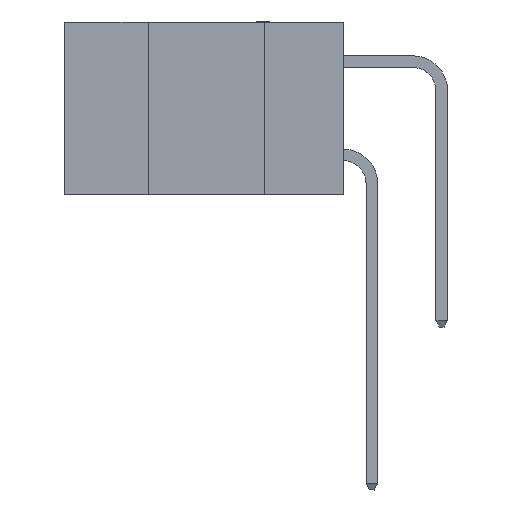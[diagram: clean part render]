
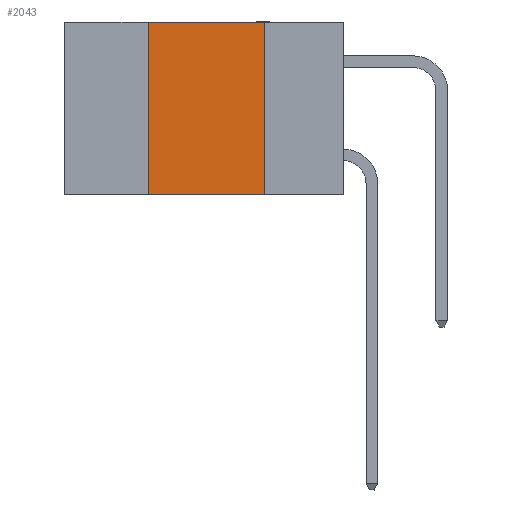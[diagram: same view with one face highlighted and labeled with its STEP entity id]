
A CAD part, left-side view. The second image highlights one B-rep face of the part: STEP entity #2043.
In plain terms, the highlighted planar face has unit normal (-1, 0, 0).
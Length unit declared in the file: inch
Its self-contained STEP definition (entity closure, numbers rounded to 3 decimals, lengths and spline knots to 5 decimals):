
#1115 = ORIENTED_EDGE ( 'NONE', *, *, #20038, .T. ) ;
#1782 = VECTOR ( 'NONE', #17318, 39.37008 ) ;
#2043 = ADVANCED_FACE ( 'NONE', ( #27690 ), #28479, .F. ) ;
#3491 = EDGE_CURVE ( 'NONE', #28054, #3561, #6715, .T. ) ;
#3561 = VERTEX_POINT ( 'NONE', #16564 ) ;
#5128 = VECTOR ( 'NONE', #19442, 39.37008 ) ;
#5188 = CARTESIAN_POINT ( 'NONE',  ( 0., 0.42, 0. ) ) ;
#5946 = DIRECTION ( 'NONE',  ( 0., 0., -1. ) ) ;
#6048 = DIRECTION ( 'NONE',  ( 1., 0., 0. ) ) ;
#6220 = DIRECTION ( 'NONE',  ( 0., -1., 0. ) ) ;
#6502 = VECTOR ( 'NONE', #22907, 39.37008 ) ;
#6715 = LINE ( 'NONE', #16647, #5128 ) ;
#7099 = ORIENTED_EDGE ( 'NONE', *, *, #25659, .F. ) ;
#7152 = EDGE_CURVE ( 'NONE', #8674, #28054, #12431, .T. ) ;
#8064 = EDGE_LOOP ( 'NONE', ( #23703, #15429, #7099, #1115 ) ) ;
#8310 = CARTESIAN_POINT ( 'NONE',  ( 0., 0.6, 0. ) ) ;
#8674 = VERTEX_POINT ( 'NONE', #5188 ) ;
#9336 = LINE ( 'NONE', #9803, #1782 ) ;
#9803 = CARTESIAN_POINT ( 'NONE',  ( 0., 0.42, 0. ) ) ;
#12431 = LINE ( 'NONE', #27914, #6502 ) ;
#15429 = ORIENTED_EDGE ( 'NONE', *, *, #7152, .F. ) ;
#16564 = CARTESIAN_POINT ( 'NONE',  ( 0., 0.17, -0.37 ) ) ;
#16647 = CARTESIAN_POINT ( 'NONE',  ( 0., 0.17, 0. ) ) ;
#17188 = LINE ( 'NONE', #28786, #23104 ) ;
#17318 = DIRECTION ( 'NONE',  ( 0., 0., 1. ) ) ;
#17916 = CARTESIAN_POINT ( 'NONE',  ( 0., 0.42, -0.37 ) ) ;
#19442 = DIRECTION ( 'NONE',  ( 0., 0., -1. ) ) ;
#19630 = CARTESIAN_POINT ( 'NONE',  ( 0., 0.17, 0. ) ) ;
#20038 = EDGE_CURVE ( 'NONE', #31365, #3561, #17188, .T. ) ;
#22907 = DIRECTION ( 'NONE',  ( 0., -1., 0. ) ) ;
#23104 = VECTOR ( 'NONE', #6220, 39.37008 ) ;
#23703 = ORIENTED_EDGE ( 'NONE', *, *, #3491, .F. ) ;
#25659 = EDGE_CURVE ( 'NONE', #31365, #8674, #9336, .T. ) ;
#26782 = AXIS2_PLACEMENT_3D ( 'NONE', #8310, #6048, #5946 ) ;
#27690 = FACE_OUTER_BOUND ( 'NONE', #8064, .T. ) ;
#27914 = CARTESIAN_POINT ( 'NONE',  ( 0., 0.6, 0. ) ) ;
#28054 = VERTEX_POINT ( 'NONE', #19630 ) ;
#28479 = PLANE ( 'NONE',  #26782 ) ;
#28786 = CARTESIAN_POINT ( 'NONE',  ( 0., 0.6, -0.37 ) ) ;
#31365 = VERTEX_POINT ( 'NONE', #17916 ) ;
